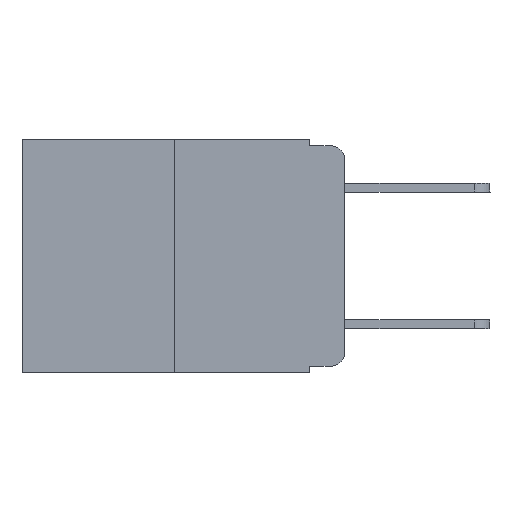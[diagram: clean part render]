
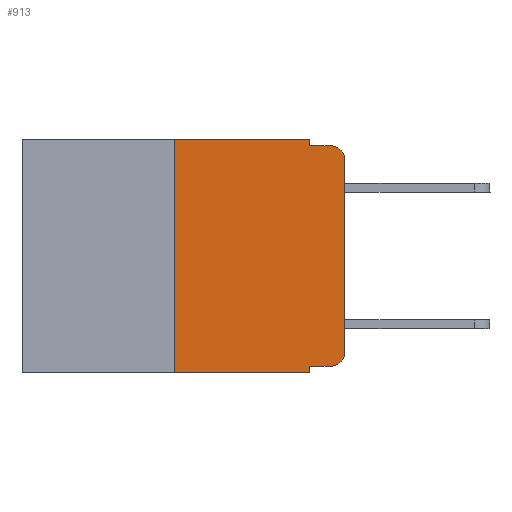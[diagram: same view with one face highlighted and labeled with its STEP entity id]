
A CAD part, left-side view. The second image highlights one B-rep face of the part: STEP entity #913.
In plain terms, the highlighted planar face has unit normal (-1, 0, 0).
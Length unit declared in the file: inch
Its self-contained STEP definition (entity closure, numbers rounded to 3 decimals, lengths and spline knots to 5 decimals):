
#74 = VECTOR ( 'NONE', #4056, 39.37008 ) ;
#84 = CARTESIAN_POINT ( 'NONE',  ( 0., 0.02, -0.01 ) ) ;
#185 = CARTESIAN_POINT ( 'NONE',  ( 0., 0.051, -0.343 ) ) ;
#294 = VERTEX_POINT ( 'NONE', #7229 ) ;
#734 = ORIENTED_EDGE ( 'NONE', *, *, #3782, .T. ) ;
#738 = VERTEX_POINT ( 'NONE', #185 ) ;
#821 = EDGE_CURVE ( 'NONE', #2125, #738, #4998, .T. ) ;
#913 = ADVANCED_FACE ( 'NONE', ( #1051 ), #2081, .F. ) ;
#956 = CARTESIAN_POINT ( 'NONE',  ( 0., 0.051, 0. ) ) ;
#1051 = FACE_OUTER_BOUND ( 'NONE', #2378, .T. ) ;
#1087 = CARTESIAN_POINT ( 'NONE',  ( 0., 0.051, -0.01 ) ) ;
#1178 = CARTESIAN_POINT ( 'NONE',  ( 0., 0.02, -0.333 ) ) ;
#1258 = CARTESIAN_POINT ( 'NONE',  ( 0., 0.051, -0.01 ) ) ;
#1395 = EDGE_CURVE ( 'NONE', #294, #738, #6708, .T. ) ;
#1617 = DIRECTION ( 'NONE',  ( 0., 0., -1. ) ) ;
#1656 = VECTOR ( 'NONE', #4072, 39.37008 ) ;
#1964 = CARTESIAN_POINT ( 'NONE',  ( 0., 0.473, -0.343 ) ) ;
#1985 = EDGE_CURVE ( 'NONE', #6652, #8622, #6554, .T. ) ;
#2001 = DIRECTION ( 'NONE',  ( 0., -1., 0. ) ) ;
#2065 = LINE ( 'NONE', #3140, #1656 ) ;
#2081 = PLANE ( 'NONE',  #6720 ) ;
#2094 = EDGE_CURVE ( 'NONE', #294, #9257, #8029, .T. ) ;
#2125 = VERTEX_POINT ( 'NONE', #3481 ) ;
#2278 = CARTESIAN_POINT ( 'NONE',  ( 0., 0.25, 0. ) ) ;
#2328 = CARTESIAN_POINT ( 'NONE',  ( 0., 0.25, 0. ) ) ;
#2378 = EDGE_LOOP ( 'NONE', ( #2515, #2994, #2415, #4255, #5572, #5433, #3977, #6905, #5044, #734 ) ) ;
#2415 = ORIENTED_EDGE ( 'NONE', *, *, #9041, .F. ) ;
#2515 = ORIENTED_EDGE ( 'NONE', *, *, #9232, .T. ) ;
#2698 = LINE ( 'NONE', #10497, #8514 ) ;
#2728 = VECTOR ( 'NONE', #2001, 39.37008 ) ;
#2885 = CARTESIAN_POINT ( 'NONE',  ( 0., 0.051, 0. ) ) ;
#2994 = ORIENTED_EDGE ( 'NONE', *, *, #1985, .T. ) ;
#3008 = DIRECTION ( 'NONE',  ( 0., 0., -1. ) ) ;
#3140 = CARTESIAN_POINT ( 'NONE',  ( 0., 0., 0. ) ) ;
#3162 = DIRECTION ( 'NONE',  ( 0., -1., 0. ) ) ;
#3440 = VERTEX_POINT ( 'NONE', #1258 ) ;
#3481 = CARTESIAN_POINT ( 'NONE',  ( 0., 0.051, -0.333 ) ) ;
#3782 = EDGE_CURVE ( 'NONE', #8146, #8658, #9051, .T. ) ;
#3977 = ORIENTED_EDGE ( 'NONE', *, *, #1395, .T. ) ;
#4056 = DIRECTION ( 'NONE',  ( 0., 0., 1. ) ) ;
#4072 = DIRECTION ( 'NONE',  ( 0., 0., 1. ) ) ;
#4169 = VERTEX_POINT ( 'NONE', #8096 ) ;
#4170 = VECTOR ( 'NONE', #4636, 39.37008 ) ;
#4255 = ORIENTED_EDGE ( 'NONE', *, *, #8277, .F. ) ;
#4280 = AXIS2_PLACEMENT_3D ( 'NONE', #6680, #9959, #1617 ) ;
#4528 = VECTOR ( 'NONE', #5963, 39.37008 ) ;
#4583 = EDGE_CURVE ( 'NONE', #9257, #4169, #7978, .T. ) ;
#4636 = DIRECTION ( 'NONE',  ( 0., 0., -1. ) ) ;
#4695 = CARTESIAN_POINT ( 'NONE',  ( 0., 0.473, 0. ) ) ;
#4998 = LINE ( 'NONE', #956, #9624 ) ;
#5044 = ORIENTED_EDGE ( 'NONE', *, *, #10317, .T. ) ;
#5231 = DIRECTION ( 'NONE',  ( 0., 0., -1. ) ) ;
#5433 = ORIENTED_EDGE ( 'NONE', *, *, #2094, .F. ) ;
#5572 = ORIENTED_EDGE ( 'NONE', *, *, #4583, .F. ) ;
#5783 = CARTESIAN_POINT ( 'NONE',  ( 0., 0., -0.03 ) ) ;
#5963 = DIRECTION ( 'NONE',  ( 0., -1., 0. ) ) ;
#6309 = DIRECTION ( 'NONE',  ( 0., 0., -1. ) ) ;
#6554 = CIRCLE ( 'NONE', #10303, 0.02 ) ;
#6652 = VERTEX_POINT ( 'NONE', #5783 ) ;
#6680 = CARTESIAN_POINT ( 'NONE',  ( 0., 0.02, -0.313 ) ) ;
#6708 = LINE ( 'NONE', #1964, #8962 ) ;
#6720 = AXIS2_PLACEMENT_3D ( 'NONE', #4695, #10644, #3008 ) ;
#6905 = ORIENTED_EDGE ( 'NONE', *, *, #821, .F. ) ;
#7229 = CARTESIAN_POINT ( 'NONE',  ( 0., 0.25, -0.343 ) ) ;
#7704 = CARTESIAN_POINT ( 'NONE',  ( 0., 0., -0.313 ) ) ;
#7978 = LINE ( 'NONE', #10250, #4528 ) ;
#8029 = LINE ( 'NONE', #2278, #74 ) ;
#8096 = CARTESIAN_POINT ( 'NONE',  ( 0., 0.051, 0. ) ) ;
#8146 = VERTEX_POINT ( 'NONE', #1178 ) ;
#8277 = EDGE_CURVE ( 'NONE', #4169, #3440, #10921, .T. ) ;
#8514 = VECTOR ( 'NONE', #8924, 39.37008 ) ;
#8622 = VERTEX_POINT ( 'NONE', #84 ) ;
#8658 = VERTEX_POINT ( 'NONE', #7704 ) ;
#8924 = DIRECTION ( 'NONE',  ( 0., -1., 0. ) ) ;
#8962 = VECTOR ( 'NONE', #3162, 39.37008 ) ;
#8973 = DIRECTION ( 'NONE',  ( -1., 0., 0. ) ) ;
#9041 = EDGE_CURVE ( 'NONE', #3440, #8622, #9462, .T. ) ;
#9051 = CIRCLE ( 'NONE', #4280, 0.02 ) ;
#9232 = EDGE_CURVE ( 'NONE', #8658, #6652, #2065, .T. ) ;
#9257 = VERTEX_POINT ( 'NONE', #2328 ) ;
#9462 = LINE ( 'NONE', #1087, #2728 ) ;
#9624 = VECTOR ( 'NONE', #5231, 39.37008 ) ;
#9959 = DIRECTION ( 'NONE',  ( -1., 0., 0. ) ) ;
#10250 = CARTESIAN_POINT ( 'NONE',  ( 0., 0.473, 0. ) ) ;
#10303 = AXIS2_PLACEMENT_3D ( 'NONE', #10512, #8973, #6309 ) ;
#10317 = EDGE_CURVE ( 'NONE', #2125, #8146, #2698, .T. ) ;
#10497 = CARTESIAN_POINT ( 'NONE',  ( 0., 0.051, -0.333 ) ) ;
#10512 = CARTESIAN_POINT ( 'NONE',  ( 0., 0.02, -0.03 ) ) ;
#10644 = DIRECTION ( 'NONE',  ( 1., 0., 0. ) ) ;
#10921 = LINE ( 'NONE', #2885, #4170 ) ;
